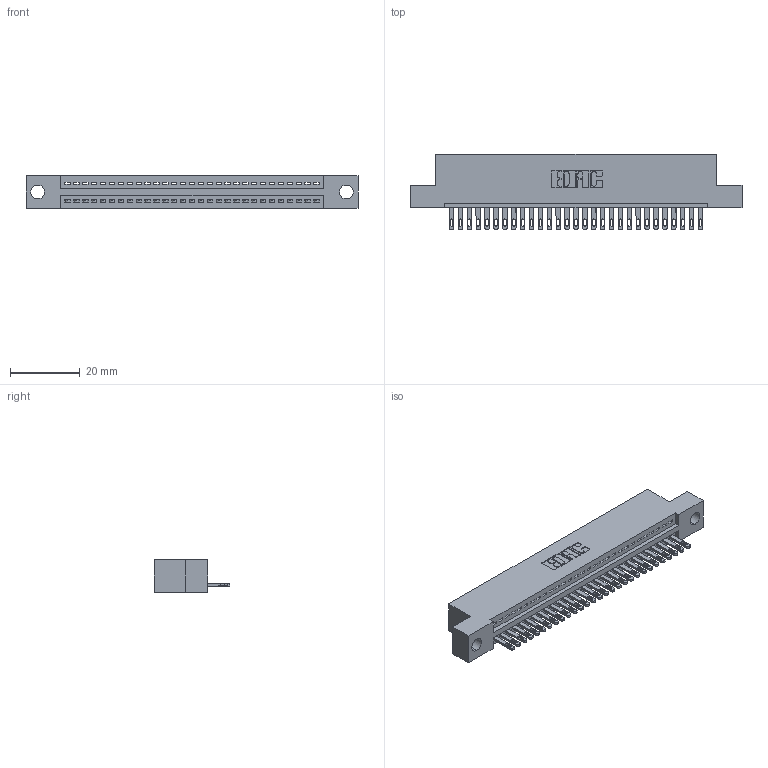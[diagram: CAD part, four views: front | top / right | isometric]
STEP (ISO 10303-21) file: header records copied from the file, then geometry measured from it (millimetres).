
FILE_DESCRIPTION (( 'STEP AP203' ), '1' );
FILE_NAME ('895-029-500-104.STEP', '2020-09-25T16:56:44', ( '' ), ( '' ), 'SwSTEP 2.0', 'SolidWorks 2020', '' );
FILE_SCHEMA (( 'CONFIG_CONTROL_DESIGN' ));
Length unit declared in the file: inch
Products named in the file (3): 345-292-001_345-293-100; 845 Part_Flush Mounting Lugs - 0.156 Dia-TH; 895-029-500-104
Assembly tree (30 placements, depth 2):
  895-029-500-104
    845 Part_Flush Mounting Lugs - 0.156 Dia-TH
    345-292-001_345-293-100  x29
Bounding box: 94.87 x 21.51 x 9.4 mm (x, y, z)
Volume: 8834.4 mm3; surface area: 11437.3 mm2
Topology: 30 solids, 30 shells, 1692 faces, 5213 edges, 3474 vertices
Faces by surface type: plane 1066, cylinder 626
Entity records: 23509 total; most frequent: CARTESIAN_POINT 4079, ORIENTED_EDGE 4042, DIRECTION 3583, EDGE_CURVE 2021, VECTOR 1769, LINE 1769, VERTEX_POINT 1346, AXIS2_PLACEMENT_3D 907
